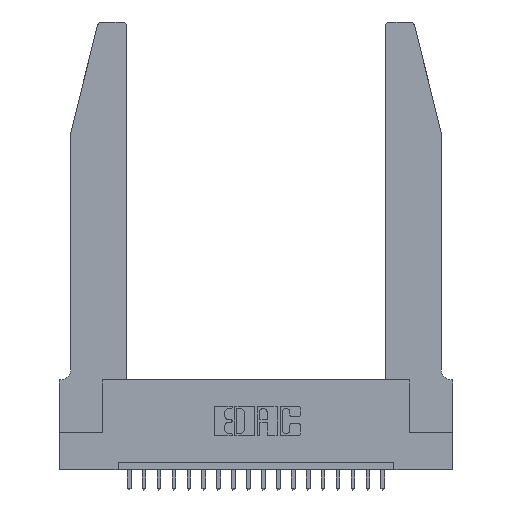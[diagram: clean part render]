
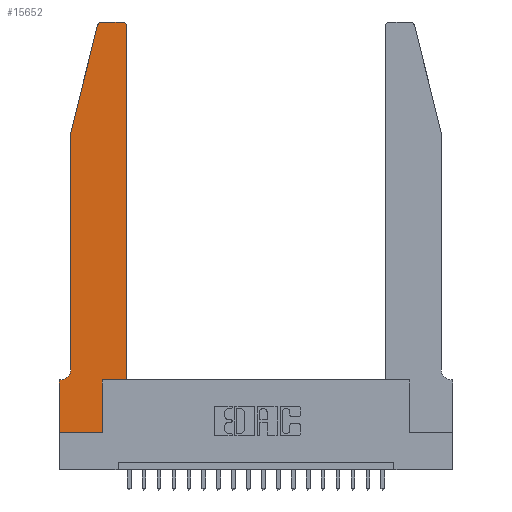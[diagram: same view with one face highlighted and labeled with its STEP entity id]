
A CAD part, top view. The second image highlights one B-rep face of the part: STEP entity #15652.
In plain terms, the highlighted planar face has unit normal (0, 0, 1).
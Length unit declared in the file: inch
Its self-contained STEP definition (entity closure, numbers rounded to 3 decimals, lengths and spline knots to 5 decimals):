
#5 = PLANE ( 'NONE',  #1558 ) ;
#111 = ORIENTED_EDGE ( 'NONE', *, *, #11465, .T. ) ;
#566 = VECTOR ( 'NONE', #18370, 39.37008 ) ;
#886 = EDGE_CURVE ( 'NONE', #5614, #18984, #13507, .T. ) ;
#1351 = CARTESIAN_POINT ( 'NONE',  ( 0.2605, 2.75, 0.37 ) ) ;
#1558 = AXIS2_PLACEMENT_3D ( 'NONE', #9989, #18508, #8454 ) ;
#1934 = ORIENTED_EDGE ( 'NONE', *, *, #14423, .T. ) ;
#2338 = EDGE_CURVE ( 'NONE', #14909, #15006, #17608, .T. ) ;
#2528 = EDGE_CURVE ( 'NONE', #15255, #13540, #7443, .T. ) ;
#3180 = CARTESIAN_POINT ( 'NONE',  ( 0.4505, 0.35, 0.37 ) ) ;
#3533 = ORIENTED_EDGE ( 'NONE', *, *, #17290, .T. ) ;
#3634 = EDGE_CURVE ( 'NONE', #11479, #5614, #10269, .T. ) ;
#3656 = CARTESIAN_POINT ( 'NONE',  ( 0., 0., 0.37 ) ) ;
#3997 = CARTESIAN_POINT ( 'NONE',  ( 0., 0., 0.37 ) ) ;
#4070 = ORIENTED_EDGE ( 'NONE', *, *, #2338, .T. ) ;
#4459 = EDGE_CURVE ( 'NONE', #20727, #14689, #9726, .T. ) ;
#4518 = CARTESIAN_POINT ( 'NONE',  ( 0.0755, 2., 0.37 ) ) ;
#4615 = EDGE_LOOP ( 'NONE', ( #17277, #20655, #6747, #5269, #111, #14728, #9524, #18236, #1934, #3533, #11731, #4070 ) ) ;
#5208 = VECTOR ( 'NONE', #13085, 39.37008 ) ;
#5269 = ORIENTED_EDGE ( 'NONE', *, *, #17719, .T. ) ;
#5564 = VECTOR ( 'NONE', #14805, 39.37008 ) ;
#5614 = VERTEX_POINT ( 'NONE', #13435 ) ;
#5889 = DIRECTION ( 'NONE',  ( 1., 0., 0. ) ) ;
#6107 = CARTESIAN_POINT ( 'NONE',  ( 0.284, 2.75, 0.37 ) ) ;
#6277 = LINE ( 'NONE', #3997, #566 ) ;
#6343 = CARTESIAN_POINT ( 'NONE',  ( 0.4505, 0.35, 0.37 ) ) ;
#6523 = AXIS2_PLACEMENT_3D ( 'NONE', #21317, #11236, #14601 ) ;
#6747 = ORIENTED_EDGE ( 'NONE', *, *, #886, .T. ) ;
#6886 = DIRECTION ( 'NONE',  ( 1., 0., 0. ) ) ;
#7059 = LINE ( 'NONE', #1351, #10953 ) ;
#7443 = LINE ( 'NONE', #8567, #21536 ) ;
#7484 = LINE ( 'NONE', #14510, #21070 ) ;
#8454 = DIRECTION ( 'NONE',  ( 1., 0., 0. ) ) ;
#8567 = CARTESIAN_POINT ( 'NONE',  ( 0.0755, 0.35, 0.37 ) ) ;
#8891 = CIRCLE ( 'NONE', #6523, 0.07 ) ;
#8973 = CARTESIAN_POINT ( 'NONE',  ( 0.4205, 2.72, 0.37 ) ) ;
#9138 = VERTEX_POINT ( 'NONE', #9477 ) ;
#9315 = VECTOR ( 'NONE', #16139, 39.37008 ) ;
#9477 = CARTESIAN_POINT ( 'NONE',  ( 0.0755, 0.42, 0.37 ) ) ;
#9524 = ORIENTED_EDGE ( 'NONE', *, *, #21041, .T. ) ;
#9696 = DIRECTION ( 'NONE',  ( -1., 0., 0. ) ) ;
#9726 = LINE ( 'NONE', #3656, #21481 ) ;
#9989 = CARTESIAN_POINT ( 'NONE',  ( 0., 0.35, 0.37 ) ) ;
#10269 = CIRCLE ( 'NONE', #13027, 0.03 ) ;
#10695 = DIRECTION ( 'NONE',  ( 1., 0., 0. ) ) ;
#10725 = DIRECTION ( 'NONE',  ( 0., 0., 1. ) ) ;
#10750 = VECTOR ( 'NONE', #18932, 39.37008 ) ;
#10801 = CARTESIAN_POINT ( 'NONE',  ( 0.0055, 0.35, 0.37 ) ) ;
#10897 = CARTESIAN_POINT ( 'NONE',  ( 0.284, 2.72, 0.37 ) ) ;
#10953 = VECTOR ( 'NONE', #9696, 39.37008 ) ;
#10985 = LINE ( 'NONE', #3180, #5564 ) ;
#11236 = DIRECTION ( 'NONE',  ( 0., 0., -1. ) ) ;
#11465 = EDGE_CURVE ( 'NONE', #9138, #15255, #8891, .T. ) ;
#11479 = VERTEX_POINT ( 'NONE', #6107 ) ;
#11731 = ORIENTED_EDGE ( 'NONE', *, *, #20293, .T. ) ;
#11892 = CARTESIAN_POINT ( 'NONE',  ( 0.0755, 2., 0.37 ) ) ;
#12041 = CARTESIAN_POINT ( 'NONE',  ( 0.4505, 0.35, 0.37 ) ) ;
#13027 = AXIS2_PLACEMENT_3D ( 'NONE', #10897, #15941, #10695 ) ;
#13078 = CARTESIAN_POINT ( 'NONE',  ( 0.4205, 2.75, 0.37 ) ) ;
#13085 = DIRECTION ( 'NONE',  ( 0., 1., 0. ) ) ;
#13435 = CARTESIAN_POINT ( 'NONE',  ( 0.25487, 2.72718, 0.37 ) ) ;
#13507 = LINE ( 'NONE', #4518, #9315 ) ;
#13540 = VERTEX_POINT ( 'NONE', #20272 ) ;
#13602 = VERTEX_POINT ( 'NONE', #12041 ) ;
#14423 = EDGE_CURVE ( 'NONE', #14689, #21120, #7484, .T. ) ;
#14510 = CARTESIAN_POINT ( 'NONE',  ( 0.2865, 0.35, 0.37 ) ) ;
#14601 = DIRECTION ( 'NONE',  ( -1., 0., 0. ) ) ;
#14689 = VERTEX_POINT ( 'NONE', #15507 ) ;
#14728 = ORIENTED_EDGE ( 'NONE', *, *, #2528, .T. ) ;
#14804 = DIRECTION ( 'NONE',  ( 0., 1., 0. ) ) ;
#14805 = DIRECTION ( 'NONE',  ( 1., 0., 0. ) ) ;
#14909 = VERTEX_POINT ( 'NONE', #16207 ) ;
#15006 = VERTEX_POINT ( 'NONE', #13078 ) ;
#15181 = LINE ( 'NONE', #15662, #10750 ) ;
#15255 = VERTEX_POINT ( 'NONE', #10801 ) ;
#15507 = CARTESIAN_POINT ( 'NONE',  ( 0.2865, 0., 0.37 ) ) ;
#15643 = CARTESIAN_POINT ( 'NONE',  ( 0., 0., 0.37 ) ) ;
#15652 = ADVANCED_FACE ( 'NONE', ( #20722 ), #5, .T. ) ;
#15662 = CARTESIAN_POINT ( 'NONE',  ( 0.0755, 2., 0.37 ) ) ;
#15852 = LINE ( 'NONE', #6343, #5208 ) ;
#15941 = DIRECTION ( 'NONE',  ( 0., 0., 1. ) ) ;
#16139 = DIRECTION ( 'NONE',  ( -0.239, -0.971, 0. ) ) ;
#16207 = CARTESIAN_POINT ( 'NONE',  ( 0.4505, 2.72, 0.37 ) ) ;
#16670 = DIRECTION ( 'NONE',  ( -1., 0., 0. ) ) ;
#16935 = AXIS2_PLACEMENT_3D ( 'NONE', #8973, #10725, #5889 ) ;
#17277 = ORIENTED_EDGE ( 'NONE', *, *, #19160, .T. ) ;
#17290 = EDGE_CURVE ( 'NONE', #21120, #13602, #10985, .T. ) ;
#17608 = CIRCLE ( 'NONE', #16935, 0.03 ) ;
#17719 = EDGE_CURVE ( 'NONE', #18984, #9138, #15181, .T. ) ;
#18236 = ORIENTED_EDGE ( 'NONE', *, *, #4459, .T. ) ;
#18370 = DIRECTION ( 'NONE',  ( 0., -1., 0. ) ) ;
#18508 = DIRECTION ( 'NONE',  ( 0., 0., 1. ) ) ;
#18932 = DIRECTION ( 'NONE',  ( 0., -1., 0. ) ) ;
#18984 = VERTEX_POINT ( 'NONE', #11892 ) ;
#19160 = EDGE_CURVE ( 'NONE', #15006, #11479, #7059, .T. ) ;
#20272 = CARTESIAN_POINT ( 'NONE',  ( 0., 0.35, 0.37 ) ) ;
#20293 = EDGE_CURVE ( 'NONE', #13602, #14909, #15852, .T. ) ;
#20655 = ORIENTED_EDGE ( 'NONE', *, *, #3634, .T. ) ;
#20722 = FACE_OUTER_BOUND ( 'NONE', #4615, .T. ) ;
#20727 = VERTEX_POINT ( 'NONE', #15643 ) ;
#20858 = CARTESIAN_POINT ( 'NONE',  ( 0.2865, 0.35, 0.37 ) ) ;
#21041 = EDGE_CURVE ( 'NONE', #13540, #20727, #6277, .T. ) ;
#21070 = VECTOR ( 'NONE', #14804, 39.37008 ) ;
#21120 = VERTEX_POINT ( 'NONE', #20858 ) ;
#21317 = CARTESIAN_POINT ( 'NONE',  ( 0.0055, 0.42, 0.37 ) ) ;
#21481 = VECTOR ( 'NONE', #6886, 39.37008 ) ;
#21536 = VECTOR ( 'NONE', #16670, 39.37008 ) ;
